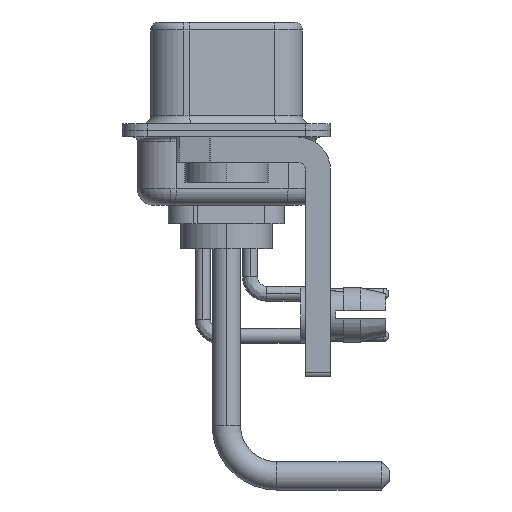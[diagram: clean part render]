
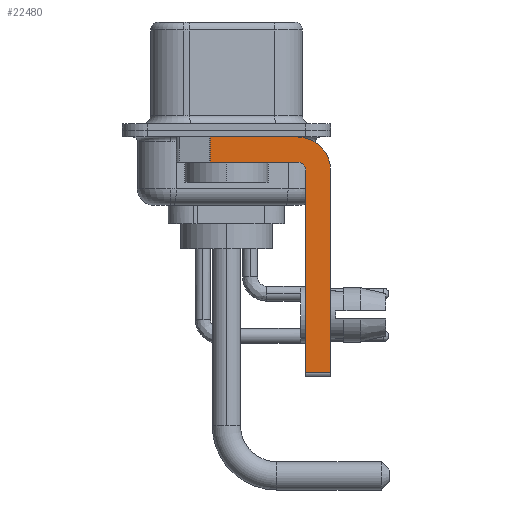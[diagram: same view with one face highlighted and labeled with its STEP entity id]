
A CAD part, left-side view. The second image highlights one B-rep face of the part: STEP entity #22480.
In plain terms, the highlighted planar face has unit normal (-1, 0, 0).
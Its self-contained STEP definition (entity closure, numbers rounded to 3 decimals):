
#131 = EDGE_CURVE ( 'NONE', #12227, #7373, #8536, .T. ) ;
#451 = CARTESIAN_POINT ( 'NONE',  ( -2.9, 0.978, -0.4 ) ) ;
#702 = VECTOR ( 'NONE', #23943, 1000. ) ;
#1108 = EDGE_CURVE ( 'NONE', #10842, #9144, #3002, .T. ) ;
#1339 = CARTESIAN_POINT ( 'NONE',  ( -2.9, -4.25, -1.9 ) ) ;
#1355 = EDGE_CURVE ( 'NONE', #25799, #14359, #19542, .T. ) ;
#1616 = AXIS2_PLACEMENT_3D ( 'NONE', #3896, #19926, #11716 ) ;
#1883 = DIRECTION ( 'NONE',  ( -1., 0., 0. ) ) ;
#2074 = ORIENTED_EDGE ( 'NONE', *, *, #1108, .F. ) ;
#3002 = LINE ( 'NONE', #21540, #6997 ) ;
#3052 = FACE_OUTER_BOUND ( 'NONE', #12668, .T. ) ;
#3182 = EDGE_CURVE ( 'NONE', #5993, #25799, #15186, .T. ) ;
#3600 = LINE ( 'NONE', #23713, #8857 ) ;
#3612 = EDGE_CURVE ( 'NONE', #10842, #14359, #3600, .T. ) ;
#3763 = CARTESIAN_POINT ( 'NONE',  ( -2.9, -4.25, -0.4 ) ) ;
#3896 = CARTESIAN_POINT ( 'NONE',  ( -2.9, -4.25, -2.4 ) ) ;
#5178 = DIRECTION ( 'NONE',  ( 1., 0., 0. ) ) ;
#5825 = CARTESIAN_POINT ( 'NONE',  ( -2.9, 3., -0.4 ) ) ;
#5993 = VERTEX_POINT ( 'NONE', #3763 ) ;
#6437 = CARTESIAN_POINT ( 'NONE',  ( -2.9, -6.25, -14.55 ) ) ;
#6449 = VECTOR ( 'NONE', #16598, 1000. ) ;
#6997 = VECTOR ( 'NONE', #25493, 1000. ) ;
#7315 = DIRECTION ( 'NONE',  ( 0., 1., 0. ) ) ;
#7367 = ORIENTED_EDGE ( 'NONE', *, *, #16642, .F. ) ;
#7373 = VERTEX_POINT ( 'NONE', #22158 ) ;
#8253 = CARTESIAN_POINT ( 'NONE',  ( -2.9, -4.75, -14.55 ) ) ;
#8536 = LINE ( 'NONE', #8805, #6449 ) ;
#8805 = CARTESIAN_POINT ( 'NONE',  ( -2.9, 0.978, -1.9 ) ) ;
#8857 = VECTOR ( 'NONE', #13673, 1000. ) ;
#9144 = VERTEX_POINT ( 'NONE', #17335 ) ;
#9625 = ORIENTED_EDGE ( 'NONE', *, *, #131, .T. ) ;
#10842 = VERTEX_POINT ( 'NONE', #8253 ) ;
#11142 = PLANE ( 'NONE',  #22227 ) ;
#11716 = DIRECTION ( 'NONE',  ( 0., 0., -1. ) ) ;
#12082 = DIRECTION ( 'NONE',  ( 0., 0., 1. ) ) ;
#12227 = VERTEX_POINT ( 'NONE', #451 ) ;
#12668 = EDGE_LOOP ( 'NONE', ( #19371, #9625, #7367, #22185, #2074, #21303, #20958, #16655 ) ) ;
#13407 = AXIS2_PLACEMENT_3D ( 'NONE', #22135, #1883, #12082 ) ;
#13673 = DIRECTION ( 'NONE',  ( 0., -1., 0. ) ) ;
#14359 = VERTEX_POINT ( 'NONE', #6437 ) ;
#15186 = CIRCLE ( 'NONE', #1616, 2. ) ;
#15244 = CARTESIAN_POINT ( 'NONE',  ( -2.9, -4.25, -2.4 ) ) ;
#15441 = VERTEX_POINT ( 'NONE', #25307 ) ;
#16598 = DIRECTION ( 'NONE',  ( 0., 0., -1. ) ) ;
#16642 = EDGE_CURVE ( 'NONE', #15441, #7373, #23980, .T. ) ;
#16655 = ORIENTED_EDGE ( 'NONE', *, *, #3182, .F. ) ;
#17335 = CARTESIAN_POINT ( 'NONE',  ( -2.9, -4.75, -2.4 ) ) ;
#17961 = CARTESIAN_POINT ( 'NONE',  ( -2.9, -6.25, -2.4 ) ) ;
#18482 = CIRCLE ( 'NONE', #13407, 0.5 ) ;
#19371 = ORIENTED_EDGE ( 'NONE', *, *, #25364, .F. ) ;
#19484 = EDGE_CURVE ( 'NONE', #9144, #15441, #18482, .T. ) ;
#19542 = LINE ( 'NONE', #17961, #24731 ) ;
#19926 = DIRECTION ( 'NONE',  ( 1., 0., 0. ) ) ;
#20108 = LINE ( 'NONE', #5825, #702 ) ;
#20958 = ORIENTED_EDGE ( 'NONE', *, *, #1355, .F. ) ;
#21303 = ORIENTED_EDGE ( 'NONE', *, *, #3612, .T. ) ;
#21327 = DIRECTION ( 'NONE',  ( 0., 0., -1. ) ) ;
#21540 = CARTESIAN_POINT ( 'NONE',  ( -2.9, -4.75, -14.8 ) ) ;
#22135 = CARTESIAN_POINT ( 'NONE',  ( -2.9, -4.25, -2.4 ) ) ;
#22158 = CARTESIAN_POINT ( 'NONE',  ( -2.9, 0.978, -1.9 ) ) ;
#22185 = ORIENTED_EDGE ( 'NONE', *, *, #19484, .F. ) ;
#22227 = AXIS2_PLACEMENT_3D ( 'NONE', #15244, #5178, #21327 ) ;
#22480 = ADVANCED_FACE ( 'NONE', ( #3052 ), #11142, .F. ) ;
#23713 = CARTESIAN_POINT ( 'NONE',  ( -2.9, -4.25, -14.55 ) ) ;
#23923 = VECTOR ( 'NONE', #7315, 1000. ) ;
#23943 = DIRECTION ( 'NONE',  ( 0., -1., 0. ) ) ;
#23980 = LINE ( 'NONE', #1339, #23923 ) ;
#24163 = CARTESIAN_POINT ( 'NONE',  ( -2.9, -6.25, -2.4 ) ) ;
#24731 = VECTOR ( 'NONE', #26148, 1000. ) ;
#25307 = CARTESIAN_POINT ( 'NONE',  ( -2.9, -4.25, -1.9 ) ) ;
#25364 = EDGE_CURVE ( 'NONE', #12227, #5993, #20108, .T. ) ;
#25493 = DIRECTION ( 'NONE',  ( 0., 0., 1. ) ) ;
#25799 = VERTEX_POINT ( 'NONE', #24163 ) ;
#26148 = DIRECTION ( 'NONE',  ( 0., 0., -1. ) ) ;
